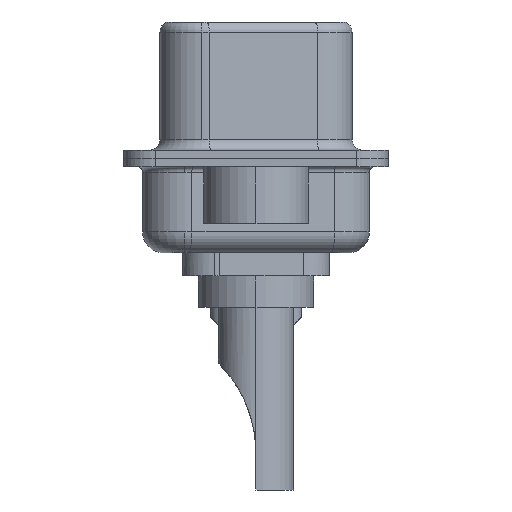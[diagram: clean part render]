
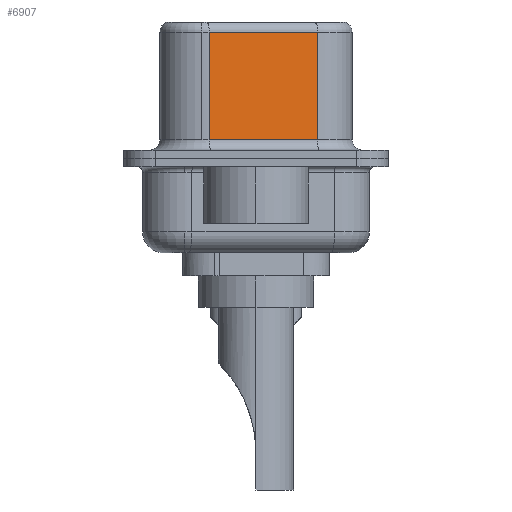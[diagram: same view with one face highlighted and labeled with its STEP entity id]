
A CAD part, left-side view. The second image highlights one B-rep face of the part: STEP entity #6907.
In plain terms, the highlighted planar face has unit normal (-0.985, -0.174, 0).
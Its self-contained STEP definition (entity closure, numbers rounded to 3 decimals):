
#362 = EDGE_CURVE ( 'NONE', #12577, #590, #7410, .T. ) ;
#590 = VERTEX_POINT ( 'NONE', #1699 ) ;
#759 = VECTOR ( 'NONE', #1604, 1000. ) ;
#1436 = EDGE_CURVE ( 'NONE', #2955, #3014, #12868, .T. ) ;
#1604 = DIRECTION ( 'NONE',  ( 0.174, -0.985, 0. ) ) ;
#1699 = CARTESIAN_POINT ( 'NONE',  ( 4.585, -2.927, 0.9 ) ) ;
#2955 = VERTEX_POINT ( 'NONE', #15561 ) ;
#3014 = VERTEX_POINT ( 'NONE', #13630 ) ;
#3983 = CARTESIAN_POINT ( 'NONE',  ( 3.675, 2.233, 0.9 ) ) ;
#4043 = EDGE_LOOP ( 'NONE', ( #8989, #11383, #16487, #12940 ) ) ;
#5223 = LINE ( 'NONE', #17052, #8506 ) ;
#5412 = VECTOR ( 'NONE', #11800, 1000. ) ;
#6046 = DIRECTION ( 'NONE',  ( 0., 0., -1. ) ) ;
#6103 = VECTOR ( 'NONE', #10904, 1000. ) ;
#6907 = ADVANCED_FACE ( 'NONE', ( #6997 ), #16383, .F. ) ;
#6997 = FACE_OUTER_BOUND ( 'NONE', #4043, .T. ) ;
#7410 = LINE ( 'NONE', #12967, #759 ) ;
#7598 = EDGE_CURVE ( 'NONE', #3014, #12577, #13555, .T. ) ;
#7668 = AXIS2_PLACEMENT_3D ( 'NONE', #16621, #16295, #16260 ) ;
#8506 = VECTOR ( 'NONE', #6046, 1000. ) ;
#8989 = ORIENTED_EDGE ( 'NONE', *, *, #13343, .F. ) ;
#10904 = DIRECTION ( 'NONE',  ( 0., 0., -1. ) ) ;
#11039 = CARTESIAN_POINT ( 'NONE',  ( 3.675, 2.233, 6.52 ) ) ;
#11383 = ORIENTED_EDGE ( 'NONE', *, *, #1436, .T. ) ;
#11800 = DIRECTION ( 'NONE',  ( -0.174, 0.985, 0. ) ) ;
#12577 = VERTEX_POINT ( 'NONE', #3983 ) ;
#12868 = LINE ( 'NONE', #14913, #5412 ) ;
#12940 = ORIENTED_EDGE ( 'NONE', *, *, #362, .T. ) ;
#12967 = CARTESIAN_POINT ( 'NONE',  ( 4.585, -2.927, 0.9 ) ) ;
#13343 = EDGE_CURVE ( 'NONE', #2955, #590, #5223, .T. ) ;
#13555 = LINE ( 'NONE', #11039, #6103 ) ;
#13630 = CARTESIAN_POINT ( 'NONE',  ( 3.675, 2.233, 6.02 ) ) ;
#14913 = CARTESIAN_POINT ( 'NONE',  ( 4.585, -2.927, 6.02 ) ) ;
#15561 = CARTESIAN_POINT ( 'NONE',  ( 4.585, -2.927, 6.02 ) ) ;
#16260 = DIRECTION ( 'NONE',  ( -0.174, 0.985, 0. ) ) ;
#16295 = DIRECTION ( 'NONE',  ( 0.985, 0.174, 0. ) ) ;
#16383 = PLANE ( 'NONE',  #7668 ) ;
#16487 = ORIENTED_EDGE ( 'NONE', *, *, #7598, .T. ) ;
#16621 = CARTESIAN_POINT ( 'NONE',  ( 4.585, -2.927, 6.52 ) ) ;
#17052 = CARTESIAN_POINT ( 'NONE',  ( 4.585, -2.927, 6.52 ) ) ;
